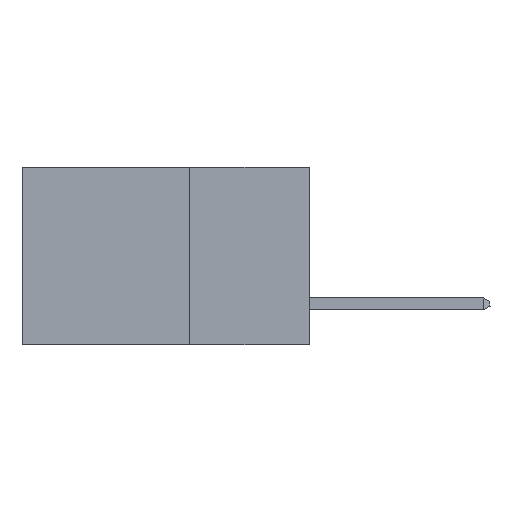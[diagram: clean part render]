
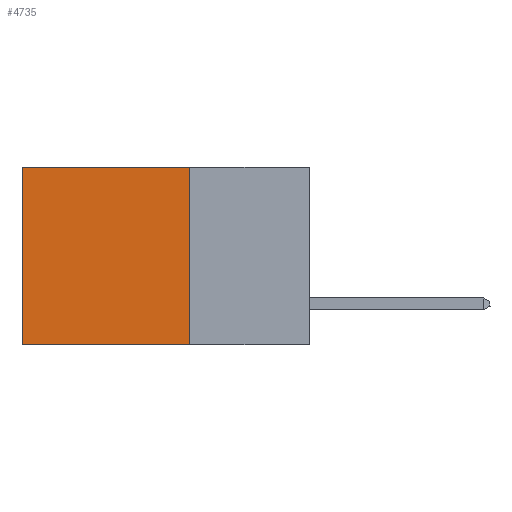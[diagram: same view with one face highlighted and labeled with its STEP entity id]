
A CAD part, left-side view. The second image highlights one B-rep face of the part: STEP entity #4735.
In plain terms, the highlighted planar face has unit normal (-1, 0, 0).
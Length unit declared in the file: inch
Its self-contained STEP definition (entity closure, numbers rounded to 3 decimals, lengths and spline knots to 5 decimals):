
#192 = ORIENTED_EDGE ( 'NONE', *, *, #4844, .F. ) ;
#382 = LINE ( 'NONE', #12862, #3188 ) ;
#811 = VECTOR ( 'NONE', #12526, 39.37008 ) ;
#1415 = CARTESIAN_POINT ( 'NONE',  ( 0.2875, 0.25, -0.37 ) ) ;
#1830 = CARTESIAN_POINT ( 'NONE',  ( 0.2875, 0.6, 0. ) ) ;
#2586 = VERTEX_POINT ( 'NONE', #1415 ) ;
#2620 = VECTOR ( 'NONE', #5812, 39.37008 ) ;
#2664 = VERTEX_POINT ( 'NONE', #10798 ) ;
#3074 = VECTOR ( 'NONE', #4422, 39.37008 ) ;
#3188 = VECTOR ( 'NONE', #5592, 39.37008 ) ;
#3472 = PLANE ( 'NONE',  #7135 ) ;
#3498 = CARTESIAN_POINT ( 'NONE',  ( 0.2875, 0.6, 0. ) ) ;
#3531 = ORIENTED_EDGE ( 'NONE', *, *, #7933, .T. ) ;
#3561 = LINE ( 'NONE', #10862, #2620 ) ;
#4403 = ORIENTED_EDGE ( 'NONE', *, *, #6163, .T. ) ;
#4422 = DIRECTION ( 'NONE',  ( 0., 1., 0. ) ) ;
#4521 = CARTESIAN_POINT ( 'NONE',  ( 0.2875, 0.25, 0. ) ) ;
#4735 = ADVANCED_FACE ( 'NONE', ( #8622 ), #3472, .F. ) ;
#4842 = VERTEX_POINT ( 'NONE', #1830 ) ;
#4844 = EDGE_CURVE ( 'NONE', #2664, #2586, #3561, .T. ) ;
#5545 = DIRECTION ( 'NONE',  ( 1., 0., 0. ) ) ;
#5592 = DIRECTION ( 'NONE',  ( 0., 1., 0. ) ) ;
#5812 = DIRECTION ( 'NONE',  ( 0., 0., -1. ) ) ;
#6095 = LINE ( 'NONE', #6369, #3074 ) ;
#6163 = EDGE_CURVE ( 'NONE', #2664, #4842, #382, .T. ) ;
#6369 = CARTESIAN_POINT ( 'NONE',  ( 0.2875, 0.25, -0.37 ) ) ;
#6862 = CARTESIAN_POINT ( 'NONE',  ( 0.2875, 0.6, -0.37 ) ) ;
#7098 = LINE ( 'NONE', #3498, #811 ) ;
#7135 = AXIS2_PLACEMENT_3D ( 'NONE', #4521, #5545, #8421 ) ;
#7933 = EDGE_CURVE ( 'NONE', #4842, #8673, #7098, .T. ) ;
#8421 = DIRECTION ( 'NONE',  ( 0., 0., -1. ) ) ;
#8622 = FACE_OUTER_BOUND ( 'NONE', #10031, .T. ) ;
#8673 = VERTEX_POINT ( 'NONE', #6862 ) ;
#10031 = EDGE_LOOP ( 'NONE', ( #3531, #12595, #192, #4403 ) ) ;
#10541 = EDGE_CURVE ( 'NONE', #2586, #8673, #6095, .T. ) ;
#10798 = CARTESIAN_POINT ( 'NONE',  ( 0.2875, 0.25, 0. ) ) ;
#10862 = CARTESIAN_POINT ( 'NONE',  ( 0.2875, 0.25, 0. ) ) ;
#12526 = DIRECTION ( 'NONE',  ( 0., 0., -1. ) ) ;
#12595 = ORIENTED_EDGE ( 'NONE', *, *, #10541, .F. ) ;
#12862 = CARTESIAN_POINT ( 'NONE',  ( 0.2875, 0.25, 0. ) ) ;
